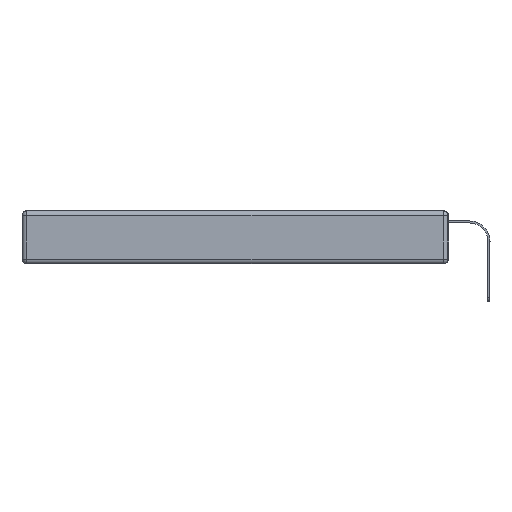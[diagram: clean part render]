
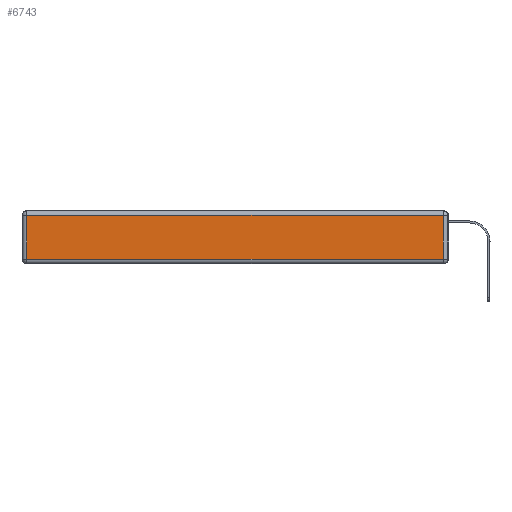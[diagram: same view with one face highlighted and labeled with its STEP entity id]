
A CAD part, left-side view. The second image highlights one B-rep face of the part: STEP entity #6743.
In plain terms, the highlighted planar face has unit normal (-1, 0, 0).
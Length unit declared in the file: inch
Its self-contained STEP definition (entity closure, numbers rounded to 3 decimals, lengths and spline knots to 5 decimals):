
#43 = VERTEX_POINT ( 'NONE', #10910 ) ;
#648 = VERTEX_POINT ( 'NONE', #12910 ) ;
#1121 = DIRECTION ( 'NONE',  ( -1., 0., 0. ) ) ;
#1136 = EDGE_CURVE ( 'NONE', #17927, #8043, #5741, .T. ) ;
#1218 = LINE ( 'NONE', #4276, #15812 ) ;
#1595 = EDGE_CURVE ( 'NONE', #43, #648, #1218, .T. ) ;
#2643 = DIRECTION ( 'NONE',  ( 0., 1., 0. ) ) ;
#3323 = EDGE_CURVE ( 'NONE', #8043, #43, #15327, .T. ) ;
#4206 = CARTESIAN_POINT ( 'NONE',  ( 0., 2.72, -0.313 ) ) ;
#4276 = CARTESIAN_POINT ( 'NONE',  ( 0., 0.03, -0.343 ) ) ;
#4385 = VECTOR ( 'NONE', #2643, 39.37008 ) ;
#4653 = EDGE_LOOP ( 'NONE', ( #15988, #9673, #10501, #17886 ) ) ;
#5244 = DIRECTION ( 'NONE',  ( 0., 0., 1. ) ) ;
#5741 = LINE ( 'NONE', #8333, #9295 ) ;
#6734 = VECTOR ( 'NONE', #16704, 39.37008 ) ;
#6743 = ADVANCED_FACE ( 'NONE', ( #15471 ), #8125, .T. ) ;
#6929 = CARTESIAN_POINT ( 'NONE',  ( 0., 2.75, -0.03 ) ) ;
#8043 = VERTEX_POINT ( 'NONE', #4206 ) ;
#8125 = PLANE ( 'NONE',  #10414 ) ;
#8333 = CARTESIAN_POINT ( 'NONE',  ( 0., 2.72, -0.343 ) ) ;
#8603 = DIRECTION ( 'NONE',  ( 0., 0., 1. ) ) ;
#9295 = VECTOR ( 'NONE', #15880, 39.37008 ) ;
#9673 = ORIENTED_EDGE ( 'NONE', *, *, #1595, .T. ) ;
#10414 = AXIS2_PLACEMENT_3D ( 'NONE', #14296, #1121, #5244 ) ;
#10501 = ORIENTED_EDGE ( 'NONE', *, *, #16972, .T. ) ;
#10910 = CARTESIAN_POINT ( 'NONE',  ( 0., 0.03, -0.313 ) ) ;
#12048 = CARTESIAN_POINT ( 'NONE',  ( 0., 2.72, -0.03 ) ) ;
#12910 = CARTESIAN_POINT ( 'NONE',  ( 0., 0.03, -0.03 ) ) ;
#14296 = CARTESIAN_POINT ( 'NONE',  ( 0., 0., -0.343 ) ) ;
#15327 = LINE ( 'NONE', #16797, #6734 ) ;
#15471 = FACE_OUTER_BOUND ( 'NONE', #4653, .T. ) ;
#15812 = VECTOR ( 'NONE', #8603, 39.37008 ) ;
#15880 = DIRECTION ( 'NONE',  ( 0., 0., -1. ) ) ;
#15988 = ORIENTED_EDGE ( 'NONE', *, *, #3323, .T. ) ;
#16704 = DIRECTION ( 'NONE',  ( 0., -1., 0. ) ) ;
#16797 = CARTESIAN_POINT ( 'NONE',  ( 0., 0., -0.313 ) ) ;
#16972 = EDGE_CURVE ( 'NONE', #648, #17927, #17375, .T. ) ;
#17375 = LINE ( 'NONE', #6929, #4385 ) ;
#17886 = ORIENTED_EDGE ( 'NONE', *, *, #1136, .T. ) ;
#17927 = VERTEX_POINT ( 'NONE', #12048 ) ;
